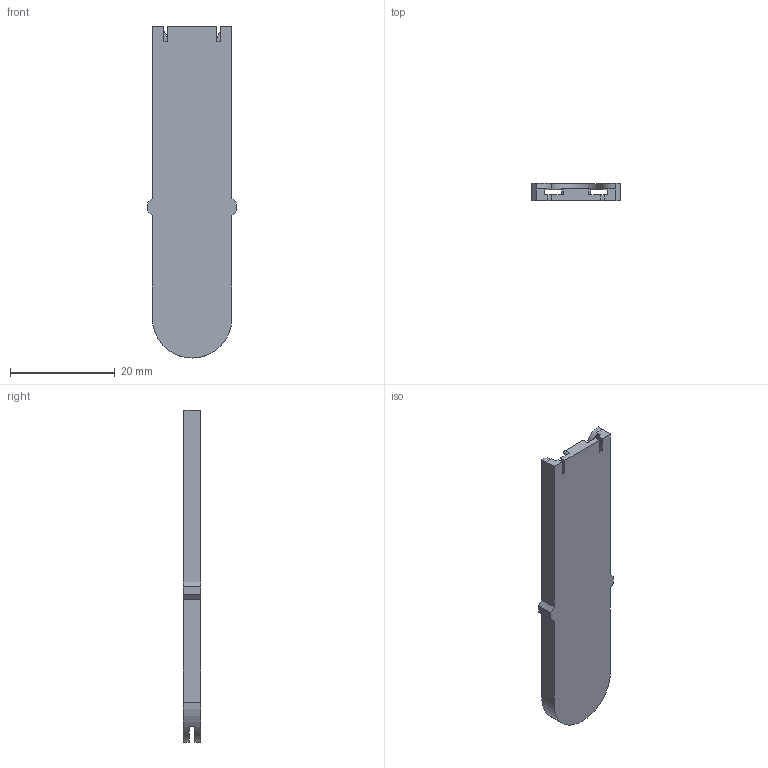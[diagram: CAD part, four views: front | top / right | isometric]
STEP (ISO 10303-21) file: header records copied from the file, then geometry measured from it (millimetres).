
FILE_DESCRIPTION (( 'STEP AP214' ), '1' );
FILE_NAME ('SKS5shotclip.STEP', '2013-08-26T13:26:37', ( 'Greg' ), ( '' ), 'SwSTEP 2.0', 'SolidWorks 2013', '' );
FILE_SCHEMA (( 'AUTOMOTIVE_DESIGN' ));
Length unit declared in the file: inch
Products named in the file (1): SKS5shotclip
Bounding box: 16.89 x 3.33 x 63.5 mm (x, y, z)
Volume: 1673.3 mm3; surface area: 3052.5 mm2
Topology: 1 solids, 1 shells, 38 faces, 110 edges, 72 vertices
Faces by surface type: plane 31, cylinder 7
Entity records: 1286 total; most frequent: CARTESIAN_POINT 221, ORIENTED_EDGE 220, DIRECTION 208, EDGE_CURVE 110, VECTOR 90, LINE 90, VERTEX_POINT 72, AXIS2_PLACEMENT_3D 59
